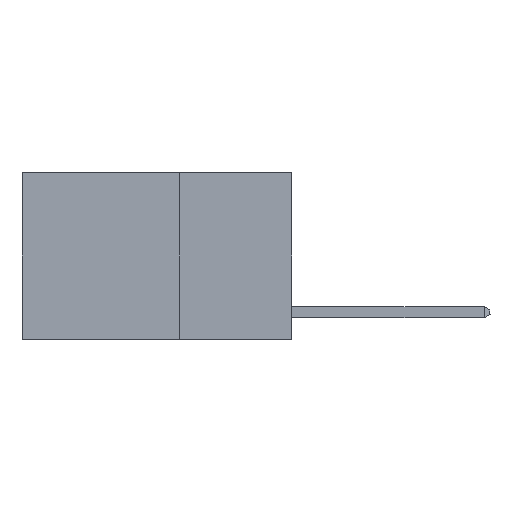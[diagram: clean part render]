
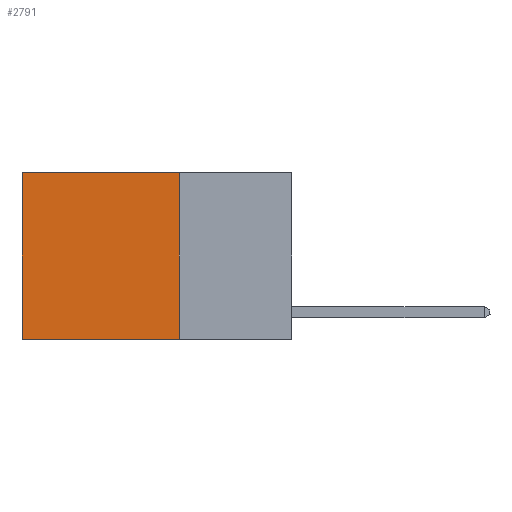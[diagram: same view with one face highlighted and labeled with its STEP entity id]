
A CAD part, left-side view. The second image highlights one B-rep face of the part: STEP entity #2791.
In plain terms, the highlighted planar face has unit normal (-1, 0, 0).
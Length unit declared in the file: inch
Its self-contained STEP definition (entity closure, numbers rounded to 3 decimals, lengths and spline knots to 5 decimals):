
#710 = VECTOR ( 'NONE', #21733, 39.37008 ) ;
#1026 = PLANE ( 'NONE',  #18538 ) ;
#1195 = ORIENTED_EDGE ( 'NONE', *, *, #14264, .F. ) ;
#1439 = LINE ( 'NONE', #15400, #3374 ) ;
#2791 = ADVANCED_FACE ( 'NONE', ( #21874 ), #1026, .F. ) ;
#3374 = VECTOR ( 'NONE', #12173, 39.37008 ) ;
#4355 = VERTEX_POINT ( 'NONE', #20956 ) ;
#4670 = VECTOR ( 'NONE', #6168, 39.37008 ) ;
#5953 = VECTOR ( 'NONE', #10570, 39.37008 ) ;
#6168 = DIRECTION ( 'NONE',  ( 0., 0., -1. ) ) ;
#6185 = DIRECTION ( 'NONE',  ( 0., 0., -1. ) ) ;
#7443 = CARTESIAN_POINT ( 'NONE',  ( 0.2625, 0.25, 0. ) ) ;
#7883 = ORIENTED_EDGE ( 'NONE', *, *, #11360, .T. ) ;
#8650 = CARTESIAN_POINT ( 'NONE',  ( 0.2625, 0.6, 0. ) ) ;
#9494 = CARTESIAN_POINT ( 'NONE',  ( 0.2625, 0.25, 0. ) ) ;
#10259 = CARTESIAN_POINT ( 'NONE',  ( 0.2625, 0.25, 0. ) ) ;
#10570 = DIRECTION ( 'NONE',  ( 0., 0., -1. ) ) ;
#10800 = ORIENTED_EDGE ( 'NONE', *, *, #22106, .F. ) ;
#10962 = LINE ( 'NONE', #7443, #4670 ) ;
#11360 = EDGE_CURVE ( 'NONE', #18051, #11674, #21841, .T. ) ;
#11603 = ORIENTED_EDGE ( 'NONE', *, *, #16118, .T. ) ;
#11674 = VERTEX_POINT ( 'NONE', #8650 ) ;
#12173 = DIRECTION ( 'NONE',  ( 0., 1., 0. ) ) ;
#13415 = EDGE_LOOP ( 'NONE', ( #11603, #1195, #10800, #7883 ) ) ;
#14264 = EDGE_CURVE ( 'NONE', #15377, #4355, #1439, .T. ) ;
#14512 = CARTESIAN_POINT ( 'NONE',  ( 0.2625, 0.25, 0. ) ) ;
#15377 = VERTEX_POINT ( 'NONE', #20238 ) ;
#15400 = CARTESIAN_POINT ( 'NONE',  ( 0.2625, 0.25, -0.37 ) ) ;
#16118 = EDGE_CURVE ( 'NONE', #11674, #4355, #19730, .T. ) ;
#17773 = CARTESIAN_POINT ( 'NONE',  ( 0.2625, 0.6, 0. ) ) ;
#18051 = VERTEX_POINT ( 'NONE', #10259 ) ;
#18538 = AXIS2_PLACEMENT_3D ( 'NONE', #9494, #21987, #6185 ) ;
#19730 = LINE ( 'NONE', #17773, #5953 ) ;
#20238 = CARTESIAN_POINT ( 'NONE',  ( 0.2625, 0.25, -0.37 ) ) ;
#20956 = CARTESIAN_POINT ( 'NONE',  ( 0.2625, 0.6, -0.37 ) ) ;
#21733 = DIRECTION ( 'NONE',  ( 0., 1., 0. ) ) ;
#21841 = LINE ( 'NONE', #14512, #710 ) ;
#21874 = FACE_OUTER_BOUND ( 'NONE', #13415, .T. ) ;
#21987 = DIRECTION ( 'NONE',  ( 1., 0., 0. ) ) ;
#22106 = EDGE_CURVE ( 'NONE', #18051, #15377, #10962, .T. ) ;
